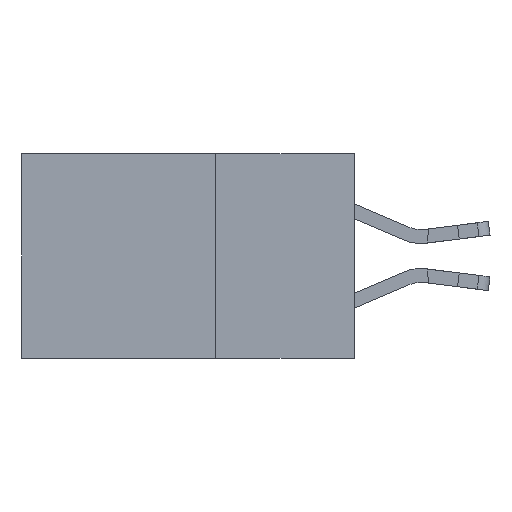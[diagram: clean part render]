
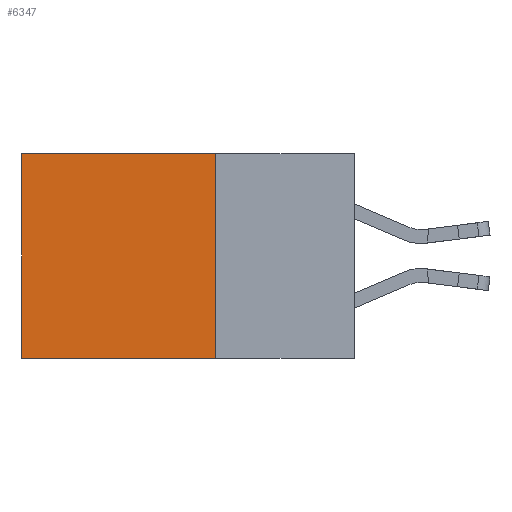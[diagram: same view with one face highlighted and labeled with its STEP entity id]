
A CAD part, left-side view. The second image highlights one B-rep face of the part: STEP entity #6347.
In plain terms, the highlighted planar face has unit normal (-1, 0, 0).
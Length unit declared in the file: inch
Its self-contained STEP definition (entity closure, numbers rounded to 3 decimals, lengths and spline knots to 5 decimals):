
#87 = VERTEX_POINT ( 'NONE', #3680 ) ;
#545 = DIRECTION ( 'NONE',  ( 0., 1., 0. ) ) ;
#746 = CARTESIAN_POINT ( 'NONE',  ( 0.298, 0.25, -0.37 ) ) ;
#1249 = VERTEX_POINT ( 'NONE', #4825 ) ;
#2462 = DIRECTION ( 'NONE',  ( 0., 0., -1. ) ) ;
#3680 = CARTESIAN_POINT ( 'NONE',  ( 0.298, 0.25, 0. ) ) ;
#3870 = CARTESIAN_POINT ( 'NONE',  ( 0.298, 0.25, 0. ) ) ;
#3874 = VECTOR ( 'NONE', #8179, 39.37008 ) ;
#4149 = FACE_OUTER_BOUND ( 'NONE', #17404, .T. ) ;
#4444 = ORIENTED_EDGE ( 'NONE', *, *, #15875, .F. ) ;
#4825 = CARTESIAN_POINT ( 'NONE',  ( 0.298, 0.6, 0. ) ) ;
#5045 = CARTESIAN_POINT ( 'NONE',  ( 0.298, 0.6, 0. ) ) ;
#5196 = ORIENTED_EDGE ( 'NONE', *, *, #19118, .F. ) ;
#6121 = CARTESIAN_POINT ( 'NONE',  ( 0.298, 0.25, -0.37 ) ) ;
#6347 = ADVANCED_FACE ( 'NONE', ( #4149 ), #16063, .F. ) ;
#6945 = LINE ( 'NONE', #3870, #14151 ) ;
#7951 = VERTEX_POINT ( 'NONE', #12552 ) ;
#8179 = DIRECTION ( 'NONE',  ( 0., 0., -1. ) ) ;
#9754 = CARTESIAN_POINT ( 'NONE',  ( 0.298, 0.25, 0. ) ) ;
#10990 = EDGE_CURVE ( 'NONE', #87, #1249, #6945, .T. ) ;
#11386 = ORIENTED_EDGE ( 'NONE', *, *, #18379, .T. ) ;
#11668 = VECTOR ( 'NONE', #545, 39.37008 ) ;
#12552 = CARTESIAN_POINT ( 'NONE',  ( 0.298, 0.6, -0.37 ) ) ;
#13483 = VECTOR ( 'NONE', #2462, 39.37008 ) ;
#13601 = LINE ( 'NONE', #746, #11668 ) ;
#14151 = VECTOR ( 'NONE', #19193, 39.37008 ) ;
#14208 = LINE ( 'NONE', #5045, #3874 ) ;
#14810 = DIRECTION ( 'NONE',  ( 0., 0., -1. ) ) ;
#15875 = EDGE_CURVE ( 'NONE', #18713, #7951, #13601, .T. ) ;
#16063 = PLANE ( 'NONE',  #18915 ) ;
#17404 = EDGE_LOOP ( 'NONE', ( #11386, #4444, #5196, #19484 ) ) ;
#17770 = CARTESIAN_POINT ( 'NONE',  ( 0.298, 0.25, 0. ) ) ;
#17905 = DIRECTION ( 'NONE',  ( 1., 0., 0. ) ) ;
#18379 = EDGE_CURVE ( 'NONE', #1249, #7951, #14208, .T. ) ;
#18713 = VERTEX_POINT ( 'NONE', #6121 ) ;
#18915 = AXIS2_PLACEMENT_3D ( 'NONE', #9754, #17905, #14810 ) ;
#19038 = LINE ( 'NONE', #17770, #13483 ) ;
#19118 = EDGE_CURVE ( 'NONE', #87, #18713, #19038, .T. ) ;
#19193 = DIRECTION ( 'NONE',  ( 0., 1., 0. ) ) ;
#19484 = ORIENTED_EDGE ( 'NONE', *, *, #10990, .T. ) ;
